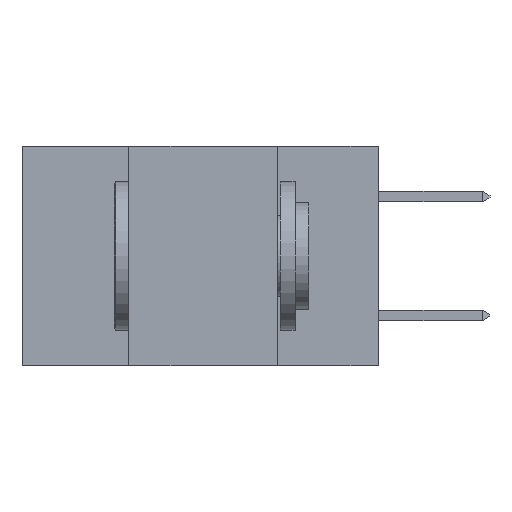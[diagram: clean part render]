
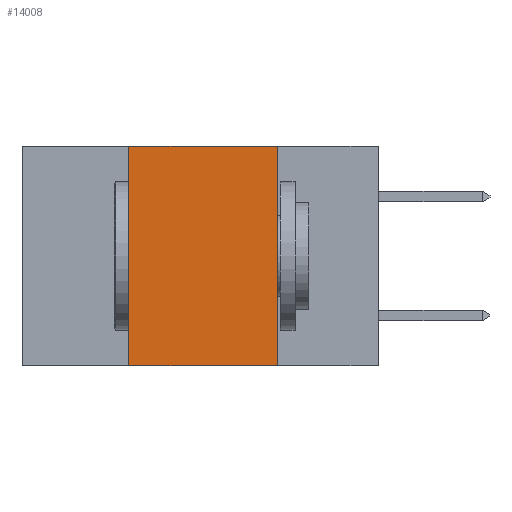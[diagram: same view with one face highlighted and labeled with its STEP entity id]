
A CAD part, left-side view. The second image highlights one B-rep face of the part: STEP entity #14008.
In plain terms, the highlighted planar face has unit normal (-1, 0, 0).
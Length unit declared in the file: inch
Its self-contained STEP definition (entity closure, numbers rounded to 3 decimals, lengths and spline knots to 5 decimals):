
#4 = FACE_OUTER_BOUND ( 'NONE', #15823, .T. ) ;
#563 = VECTOR ( 'NONE', #6894, 39.37008 ) ;
#712 = VERTEX_POINT ( 'NONE', #811 ) ;
#811 = CARTESIAN_POINT ( 'NONE',  ( 0., 0.42, -0.37 ) ) ;
#1454 = ORIENTED_EDGE ( 'NONE', *, *, #6242, .F. ) ;
#1931 = CARTESIAN_POINT ( 'NONE',  ( 0., 0.42, 0. ) ) ;
#1994 = ORIENTED_EDGE ( 'NONE', *, *, #16060, .T. ) ;
#2681 = LINE ( 'NONE', #11706, #15926 ) ;
#3198 = VECTOR ( 'NONE', #4017, 39.37008 ) ;
#4017 = DIRECTION ( 'NONE',  ( 0., -1., 0. ) ) ;
#4308 = CARTESIAN_POINT ( 'NONE',  ( 0., 0.17, 0. ) ) ;
#4981 = CARTESIAN_POINT ( 'NONE',  ( 0., 0.6, 0. ) ) ;
#6144 = LINE ( 'NONE', #14257, #3198 ) ;
#6188 = PLANE ( 'NONE',  #14908 ) ;
#6238 = DIRECTION ( 'NONE',  ( 0., 0., -1. ) ) ;
#6242 = EDGE_CURVE ( 'NONE', #13747, #16200, #2681, .T. ) ;
#6561 = DIRECTION ( 'NONE',  ( 0., -1., 0. ) ) ;
#6894 = DIRECTION ( 'NONE',  ( 0., 0., 1. ) ) ;
#8616 = VERTEX_POINT ( 'NONE', #12781 ) ;
#8760 = VECTOR ( 'NONE', #14612, 39.37008 ) ;
#9333 = ORIENTED_EDGE ( 'NONE', *, *, #14308, .F. ) ;
#10751 = LINE ( 'NONE', #15993, #563 ) ;
#11706 = CARTESIAN_POINT ( 'NONE',  ( 0., 0.6, 0. ) ) ;
#11890 = ORIENTED_EDGE ( 'NONE', *, *, #16278, .F. ) ;
#11967 = CARTESIAN_POINT ( 'NONE',  ( 0., 0.17, 0. ) ) ;
#12264 = LINE ( 'NONE', #4308, #8760 ) ;
#12781 = CARTESIAN_POINT ( 'NONE',  ( 0., 0.17, -0.37 ) ) ;
#13747 = VERTEX_POINT ( 'NONE', #1931 ) ;
#13998 = DIRECTION ( 'NONE',  ( 1., 0., 0. ) ) ;
#14008 = ADVANCED_FACE ( 'NONE', ( #4 ), #6188, .F. ) ;
#14257 = CARTESIAN_POINT ( 'NONE',  ( 0., 0.6, -0.37 ) ) ;
#14308 = EDGE_CURVE ( 'NONE', #16200, #8616, #12264, .T. ) ;
#14612 = DIRECTION ( 'NONE',  ( 0., 0., -1. ) ) ;
#14908 = AXIS2_PLACEMENT_3D ( 'NONE', #4981, #13998, #6238 ) ;
#15823 = EDGE_LOOP ( 'NONE', ( #9333, #1454, #11890, #1994 ) ) ;
#15926 = VECTOR ( 'NONE', #6561, 39.37008 ) ;
#15993 = CARTESIAN_POINT ( 'NONE',  ( 0., 0.42, 0. ) ) ;
#16060 = EDGE_CURVE ( 'NONE', #712, #8616, #6144, .T. ) ;
#16200 = VERTEX_POINT ( 'NONE', #11967 ) ;
#16278 = EDGE_CURVE ( 'NONE', #712, #13747, #10751, .T. ) ;
